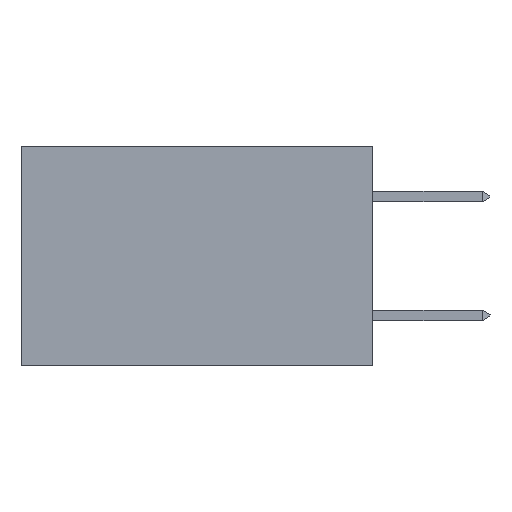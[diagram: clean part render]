
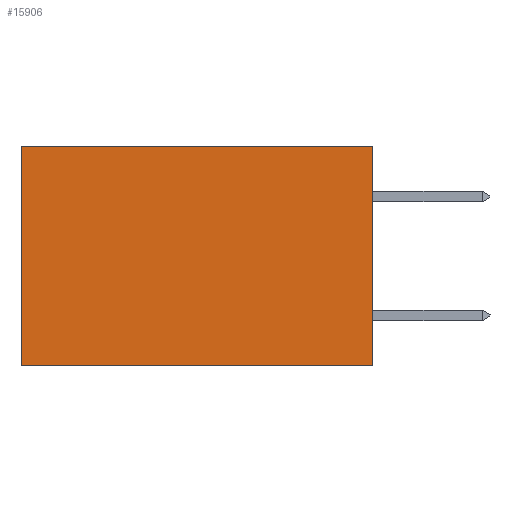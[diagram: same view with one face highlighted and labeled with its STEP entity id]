
A CAD part, left-side view. The second image highlights one B-rep face of the part: STEP entity #15906.
In plain terms, the highlighted planar face has unit normal (-1, 0, 0).
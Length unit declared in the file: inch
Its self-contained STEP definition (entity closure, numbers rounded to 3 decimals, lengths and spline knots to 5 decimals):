
#21 = VERTEX_POINT ( 'NONE', #9868 ) ;
#364 = AXIS2_PLACEMENT_3D ( 'NONE', #17329, #9349, #1083 ) ;
#717 = ORIENTED_EDGE ( 'NONE', *, *, #16053, .T. ) ;
#1083 = DIRECTION ( 'NONE',  ( 0., 0., -1. ) ) ;
#2183 = CARTESIAN_POINT ( 'NONE',  ( 0.277, 0., -0.37 ) ) ;
#2519 = VERTEX_POINT ( 'NONE', #2183 ) ;
#2718 = VERTEX_POINT ( 'NONE', #4576 ) ;
#3597 = CARTESIAN_POINT ( 'NONE',  ( 0.277, 0.59, -0.37 ) ) ;
#3822 = DIRECTION ( 'NONE',  ( 0., 1., 0. ) ) ;
#3979 = ORIENTED_EDGE ( 'NONE', *, *, #16157, .F. ) ;
#4044 = LINE ( 'NONE', #13794, #10871 ) ;
#4271 = FACE_OUTER_BOUND ( 'NONE', #12503, .T. ) ;
#4576 = CARTESIAN_POINT ( 'NONE',  ( 0.277, 0., 0. ) ) ;
#4918 = VECTOR ( 'NONE', #12277, 39.37008 ) ;
#7054 = ORIENTED_EDGE ( 'NONE', *, *, #10795, .T. ) ;
#7436 = ORIENTED_EDGE ( 'NONE', *, *, #15175, .F. ) ;
#8609 = LINE ( 'NONE', #13618, #4918 ) ;
#9349 = DIRECTION ( 'NONE',  ( 1., 0., 0. ) ) ;
#9868 = CARTESIAN_POINT ( 'NONE',  ( 0.277, 0.59, 0. ) ) ;
#10058 = VERTEX_POINT ( 'NONE', #3597 ) ;
#10292 = VECTOR ( 'NONE', #3822, 39.37008 ) ;
#10795 = EDGE_CURVE ( 'NONE', #2718, #21, #13822, .T. ) ;
#10871 = VECTOR ( 'NONE', #15165, 39.37008 ) ;
#11313 = VECTOR ( 'NONE', #16245, 39.37008 ) ;
#11698 = LINE ( 'NONE', #12169, #11313 ) ;
#11913 = PLANE ( 'NONE',  #364 ) ;
#12169 = CARTESIAN_POINT ( 'NONE',  ( 0.277, 0., -0.37 ) ) ;
#12277 = DIRECTION ( 'NONE',  ( 0., 0., -1. ) ) ;
#12503 = EDGE_LOOP ( 'NONE', ( #717, #3979, #7436, #7054 ) ) ;
#13618 = CARTESIAN_POINT ( 'NONE',  ( 0.277, 0.59, -0.37 ) ) ;
#13794 = CARTESIAN_POINT ( 'NONE',  ( 0.277, 0., -0.37 ) ) ;
#13822 = LINE ( 'NONE', #15961, #10292 ) ;
#15165 = DIRECTION ( 'NONE',  ( 0., 1., 0. ) ) ;
#15175 = EDGE_CURVE ( 'NONE', #2718, #2519, #11698, .T. ) ;
#15906 = ADVANCED_FACE ( 'NONE', ( #4271 ), #11913, .F. ) ;
#15961 = CARTESIAN_POINT ( 'NONE',  ( 0.277, 0., 0. ) ) ;
#16053 = EDGE_CURVE ( 'NONE', #21, #10058, #8609, .T. ) ;
#16157 = EDGE_CURVE ( 'NONE', #2519, #10058, #4044, .T. ) ;
#16245 = DIRECTION ( 'NONE',  ( 0., 0., -1. ) ) ;
#17329 = CARTESIAN_POINT ( 'NONE',  ( 0.277, 0., -0.37 ) ) ;
